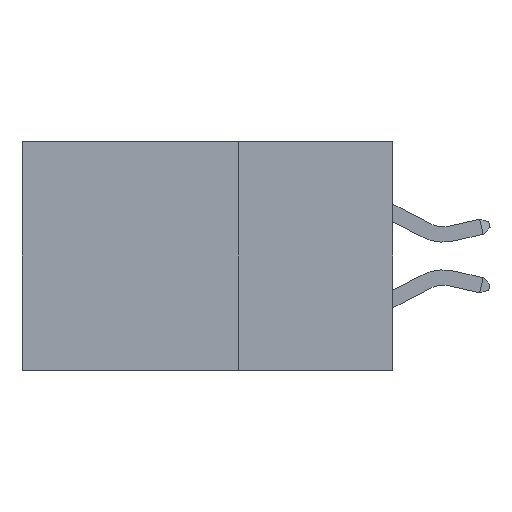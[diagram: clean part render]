
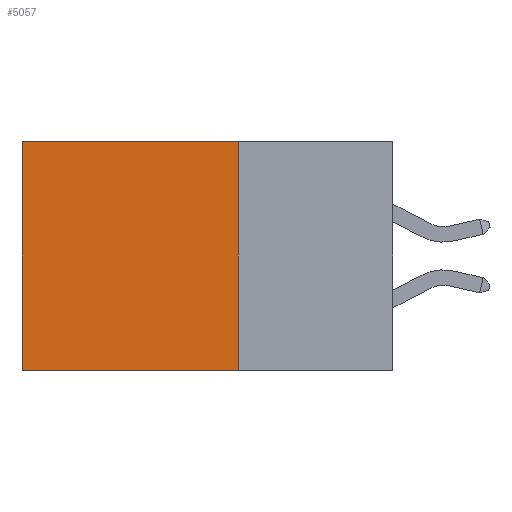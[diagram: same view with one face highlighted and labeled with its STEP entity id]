
A CAD part, left-side view. The second image highlights one B-rep face of the part: STEP entity #5057.
In plain terms, the highlighted planar face has unit normal (-1, 0, 0).
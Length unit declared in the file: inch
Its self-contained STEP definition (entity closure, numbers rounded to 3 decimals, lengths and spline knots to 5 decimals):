
#1160 = EDGE_CURVE ( 'NONE', #8764, #2800, #3572, .T. ) ;
#1198 = ORIENTED_EDGE ( 'NONE', *, *, #1160, .F. ) ;
#1302 = DIRECTION ( 'NONE',  ( 0., 0., -1. ) ) ;
#2087 = VERTEX_POINT ( 'NONE', #5762 ) ;
#2166 = EDGE_CURVE ( 'NONE', #8764, #10447, #9093, .T. ) ;
#2641 = FACE_OUTER_BOUND ( 'NONE', #3340, .T. ) ;
#2753 = CARTESIAN_POINT ( 'NONE',  ( 0.2875, 0.25, 0. ) ) ;
#2792 = CARTESIAN_POINT ( 'NONE',  ( 0.2875, 0.6, 0. ) ) ;
#2800 = VERTEX_POINT ( 'NONE', #9919 ) ;
#3340 = EDGE_LOOP ( 'NONE', ( #4137, #10198, #1198, #4865 ) ) ;
#3572 = LINE ( 'NONE', #10338, #3811 ) ;
#3811 = VECTOR ( 'NONE', #1302, 39.37008 ) ;
#4137 = ORIENTED_EDGE ( 'NONE', *, *, #5380, .T. ) ;
#4682 = DIRECTION ( 'NONE',  ( 0., 1., 0. ) ) ;
#4701 = CARTESIAN_POINT ( 'NONE',  ( 0.2875, 0.25, 0. ) ) ;
#4865 = ORIENTED_EDGE ( 'NONE', *, *, #2166, .T. ) ;
#5057 = ADVANCED_FACE ( 'NONE', ( #2641 ), #10376, .F. ) ;
#5380 = EDGE_CURVE ( 'NONE', #10447, #2087, #8160, .T. ) ;
#5762 = CARTESIAN_POINT ( 'NONE',  ( 0.2875, 0.6, -0.37 ) ) ;
#5800 = DIRECTION ( 'NONE',  ( 0., 1., 0. ) ) ;
#5833 = CARTESIAN_POINT ( 'NONE',  ( 0.2875, 0.25, -0.37 ) ) ;
#5926 = AXIS2_PLACEMENT_3D ( 'NONE', #10270, #10255, #10237 ) ;
#8160 = LINE ( 'NONE', #9036, #9798 ) ;
#8228 = VECTOR ( 'NONE', #5800, 39.37008 ) ;
#8611 = VECTOR ( 'NONE', #4682, 39.37008 ) ;
#8764 = VERTEX_POINT ( 'NONE', #2753 ) ;
#9013 = DIRECTION ( 'NONE',  ( 0., 0., -1. ) ) ;
#9036 = CARTESIAN_POINT ( 'NONE',  ( 0.2875, 0.6, 0. ) ) ;
#9093 = LINE ( 'NONE', #4701, #8611 ) ;
#9480 = EDGE_CURVE ( 'NONE', #2800, #2087, #10353, .T. ) ;
#9798 = VECTOR ( 'NONE', #9013, 39.37008 ) ;
#9919 = CARTESIAN_POINT ( 'NONE',  ( 0.2875, 0.25, -0.37 ) ) ;
#10198 = ORIENTED_EDGE ( 'NONE', *, *, #9480, .F. ) ;
#10237 = DIRECTION ( 'NONE',  ( 0., 0., -1. ) ) ;
#10255 = DIRECTION ( 'NONE',  ( 1., 0., 0. ) ) ;
#10270 = CARTESIAN_POINT ( 'NONE',  ( 0.2875, 0.25, 0. ) ) ;
#10338 = CARTESIAN_POINT ( 'NONE',  ( 0.2875, 0.25, 0. ) ) ;
#10353 = LINE ( 'NONE', #5833, #8228 ) ;
#10376 = PLANE ( 'NONE',  #5926 ) ;
#10447 = VERTEX_POINT ( 'NONE', #2792 ) ;
